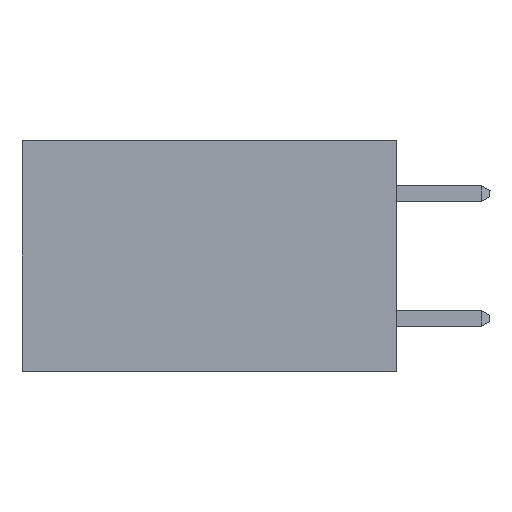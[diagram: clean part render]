
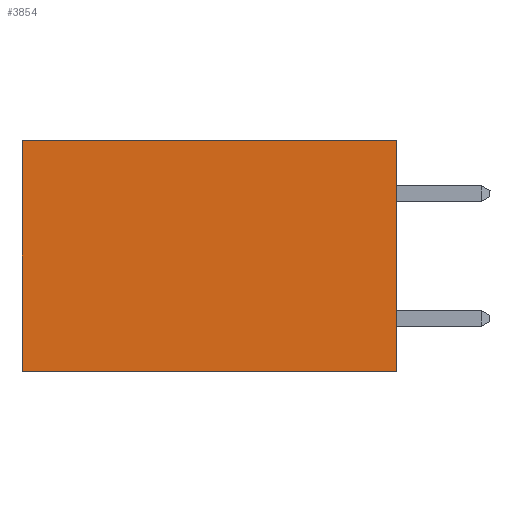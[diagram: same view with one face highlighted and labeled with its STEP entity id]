
A CAD part, left-side view. The second image highlights one B-rep face of the part: STEP entity #3854.
In plain terms, the highlighted planar face has unit normal (-1, 0, 0).
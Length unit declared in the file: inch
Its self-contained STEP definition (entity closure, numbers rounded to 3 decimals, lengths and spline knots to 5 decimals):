
#169 = CARTESIAN_POINT ( 'NONE',  ( 0.298, 0., 0. ) ) ;
#1286 = FACE_OUTER_BOUND ( 'NONE', #8351, .T. ) ;
#1843 = VERTEX_POINT ( 'NONE', #9610 ) ;
#1973 = LINE ( 'NONE', #7138, #9337 ) ;
#2041 = VERTEX_POINT ( 'NONE', #10413 ) ;
#3172 = ORIENTED_EDGE ( 'NONE', *, *, #8517, .T. ) ;
#3487 = ORIENTED_EDGE ( 'NONE', *, *, #6946, .F. ) ;
#3695 = DIRECTION ( 'NONE',  ( 0., 0., -1. ) ) ;
#3854 = ADVANCED_FACE ( 'NONE', ( #1286 ), #4272, .F. ) ;
#4272 = PLANE ( 'NONE',  #9480 ) ;
#4572 = DIRECTION ( 'NONE',  ( 1., 0., 0. ) ) ;
#5020 = VERTEX_POINT ( 'NONE', #7317 ) ;
#5063 = EDGE_CURVE ( 'NONE', #1843, #2041, #1973, .T. ) ;
#5541 = DIRECTION ( 'NONE',  ( 0., 1., 0. ) ) ;
#5695 = LINE ( 'NONE', #169, #8569 ) ;
#5726 = ORIENTED_EDGE ( 'NONE', *, *, #6754, .F. ) ;
#6754 = EDGE_CURVE ( 'NONE', #8514, #2041, #10334, .T. ) ;
#6946 = EDGE_CURVE ( 'NONE', #5020, #8514, #5695, .T. ) ;
#7138 = CARTESIAN_POINT ( 'NONE',  ( 0.298, 0.6, 0. ) ) ;
#7200 = VECTOR ( 'NONE', #11985, 39.37008 ) ;
#7317 = CARTESIAN_POINT ( 'NONE',  ( 0.298, 0., 0. ) ) ;
#7344 = DIRECTION ( 'NONE',  ( 0., 0., -1. ) ) ;
#7521 = ORIENTED_EDGE ( 'NONE', *, *, #5063, .T. ) ;
#8351 = EDGE_LOOP ( 'NONE', ( #7521, #5726, #3487, #3172 ) ) ;
#8422 = CARTESIAN_POINT ( 'NONE',  ( 0.298, 0., -0.37 ) ) ;
#8514 = VERTEX_POINT ( 'NONE', #8422 ) ;
#8517 = EDGE_CURVE ( 'NONE', #5020, #1843, #11861, .T. ) ;
#8569 = VECTOR ( 'NONE', #3695, 39.37008 ) ;
#9337 = VECTOR ( 'NONE', #7344, 39.37008 ) ;
#9423 = VECTOR ( 'NONE', #5541, 39.37008 ) ;
#9480 = AXIS2_PLACEMENT_3D ( 'NONE', #10654, #4572, #12099 ) ;
#9610 = CARTESIAN_POINT ( 'NONE',  ( 0.298, 0.6, 0. ) ) ;
#10143 = CARTESIAN_POINT ( 'NONE',  ( 0.298, 0., -0.37 ) ) ;
#10334 = LINE ( 'NONE', #10143, #7200 ) ;
#10413 = CARTESIAN_POINT ( 'NONE',  ( 0.298, 0.6, -0.37 ) ) ;
#10654 = CARTESIAN_POINT ( 'NONE',  ( 0.298, 0., 0. ) ) ;
#11229 = CARTESIAN_POINT ( 'NONE',  ( 0.298, 0., 0. ) ) ;
#11861 = LINE ( 'NONE', #11229, #9423 ) ;
#11985 = DIRECTION ( 'NONE',  ( 0., 1., 0. ) ) ;
#12099 = DIRECTION ( 'NONE',  ( 0., 0., -1. ) ) ;
